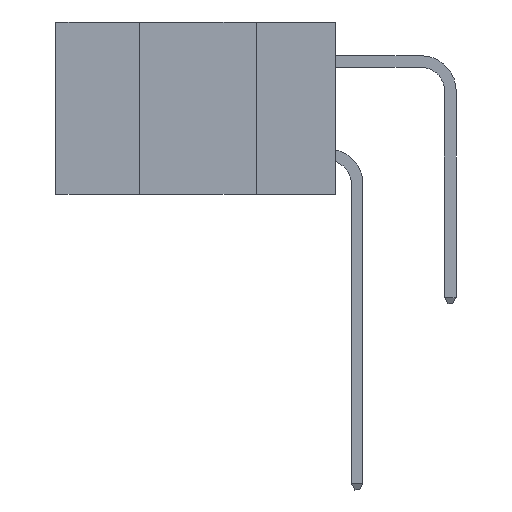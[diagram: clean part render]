
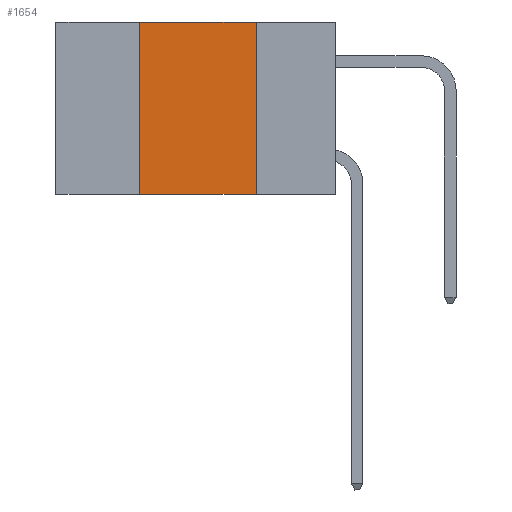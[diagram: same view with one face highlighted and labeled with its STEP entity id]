
A CAD part, left-side view. The second image highlights one B-rep face of the part: STEP entity #1654.
In plain terms, the highlighted planar face has unit normal (-1, 0, 0).
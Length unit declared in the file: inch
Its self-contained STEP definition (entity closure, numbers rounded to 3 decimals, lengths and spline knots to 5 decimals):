
#1283 = PLANE ( 'NONE',  #7328 ) ;
#1293 = EDGE_CURVE ( 'NONE', #15074, #2617, #6729, .T. ) ;
#1381 = VECTOR ( 'NONE', #4492, 39.37008 ) ;
#1654 = ADVANCED_FACE ( 'NONE', ( #9926 ), #1283, .F. ) ;
#1677 = EDGE_CURVE ( 'NONE', #15074, #7627, #2995, .T. ) ;
#1763 = CARTESIAN_POINT ( 'NONE',  ( 0., 0.6, 0. ) ) ;
#2343 = DIRECTION ( 'NONE',  ( 0., -1., 0. ) ) ;
#2617 = VERTEX_POINT ( 'NONE', #16158 ) ;
#2789 = CARTESIAN_POINT ( 'NONE',  ( 0., 0.6, 0. ) ) ;
#2995 = LINE ( 'NONE', #3411, #15510 ) ;
#3411 = CARTESIAN_POINT ( 'NONE',  ( 0., 0.42, 0. ) ) ;
#3414 = VECTOR ( 'NONE', #2343, 39.37008 ) ;
#4479 = CARTESIAN_POINT ( 'NONE',  ( 0., 0.17, 0. ) ) ;
#4492 = DIRECTION ( 'NONE',  ( 0., -1., 0. ) ) ;
#4722 = DIRECTION ( 'NONE',  ( 0., 0., -1. ) ) ;
#5154 = LINE ( 'NONE', #1763, #1381 ) ;
#5383 = DIRECTION ( 'NONE',  ( 0., 0., -1. ) ) ;
#6589 = ORIENTED_EDGE ( 'NONE', *, *, #1677, .F. ) ;
#6729 = LINE ( 'NONE', #15001, #3414 ) ;
#7328 = AXIS2_PLACEMENT_3D ( 'NONE', #2789, #11049, #4722 ) ;
#7627 = VERTEX_POINT ( 'NONE', #13177 ) ;
#7714 = VECTOR ( 'NONE', #5383, 39.37008 ) ;
#9029 = LINE ( 'NONE', #15939, #7714 ) ;
#9926 = FACE_OUTER_BOUND ( 'NONE', #10210, .T. ) ;
#10054 = EDGE_CURVE ( 'NONE', #7627, #11618, #5154, .T. ) ;
#10210 = EDGE_LOOP ( 'NONE', ( #10242, #15252, #6589, #15238 ) ) ;
#10242 = ORIENTED_EDGE ( 'NONE', *, *, #11792, .F. ) ;
#11049 = DIRECTION ( 'NONE',  ( 1., 0., 0. ) ) ;
#11618 = VERTEX_POINT ( 'NONE', #4479 ) ;
#11792 = EDGE_CURVE ( 'NONE', #11618, #2617, #9029, .T. ) ;
#12733 = DIRECTION ( 'NONE',  ( 0., 0., 1. ) ) ;
#13177 = CARTESIAN_POINT ( 'NONE',  ( 0., 0.42, 0. ) ) ;
#15001 = CARTESIAN_POINT ( 'NONE',  ( 0., 0.6, -0.37 ) ) ;
#15074 = VERTEX_POINT ( 'NONE', #16113 ) ;
#15238 = ORIENTED_EDGE ( 'NONE', *, *, #1293, .T. ) ;
#15252 = ORIENTED_EDGE ( 'NONE', *, *, #10054, .F. ) ;
#15510 = VECTOR ( 'NONE', #12733, 39.37008 ) ;
#15939 = CARTESIAN_POINT ( 'NONE',  ( 0., 0.17, 0. ) ) ;
#16113 = CARTESIAN_POINT ( 'NONE',  ( 0., 0.42, -0.37 ) ) ;
#16158 = CARTESIAN_POINT ( 'NONE',  ( 0., 0.17, -0.37 ) ) ;
